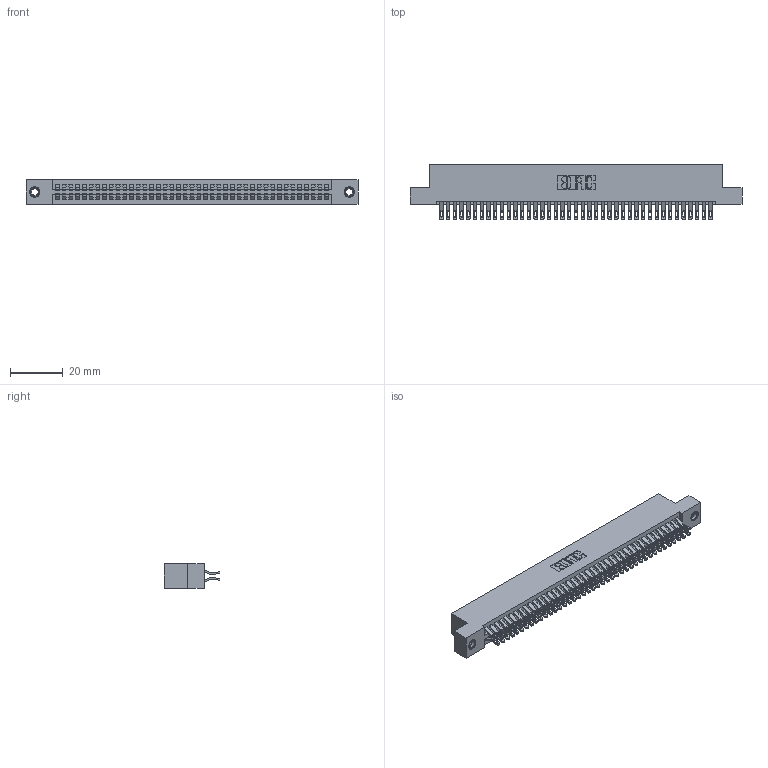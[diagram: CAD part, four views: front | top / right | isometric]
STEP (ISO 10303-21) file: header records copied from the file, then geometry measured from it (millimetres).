
FILE_DESCRIPTION (( 'STEP AP203' ), '1' );
FILE_NAME ('395-082-555-207.STEP', '2018-11-28T09:03:38', ( '' ), ( '' ), 'SwSTEP 2.0', 'SolidWorks 2016', '' );
FILE_SCHEMA (( 'CONFIG_CONTROL_DESIGN' ));
Length unit declared in the file: inch
Products named in the file (4): 395-082-555-207; 345-292-001_555 Tail; 345 Part_Flush Mounting Lugs - 0.156 Dia-TI; 345-250-001_345-250-005-103
Assembly tree (85 placements, depth 2):
  395-082-555-207
    345 Part_Flush Mounting Lugs - 0.156 Dia-TI
    345-292-001_555 Tail  x82
    345-250-001_345-250-005-103  x2
Bounding box: 125.35 x 21.13 x 9.4 mm (x, y, z)
Volume: 12391.6 mm3; surface area: 19152.6 mm2
Topology: 85 solids, 85 shells, 4778 faces, 14991 edges, 9986 vertices
Faces by surface type: plane 2654, cylinder 2108, cone 12, torus 4
Entity records: 33816 total; most frequent: CARTESIAN_POINT 5685, ORIENTED_EDGE 5582, DIRECTION 5009, EDGE_CURVE 2791, LINE 2455, VECTOR 2455, VERTEX_POINT 1856, AXIS2_PLACEMENT_3D 1277
